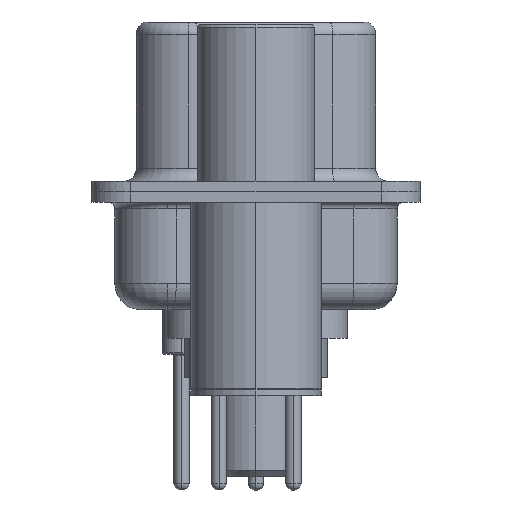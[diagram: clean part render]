
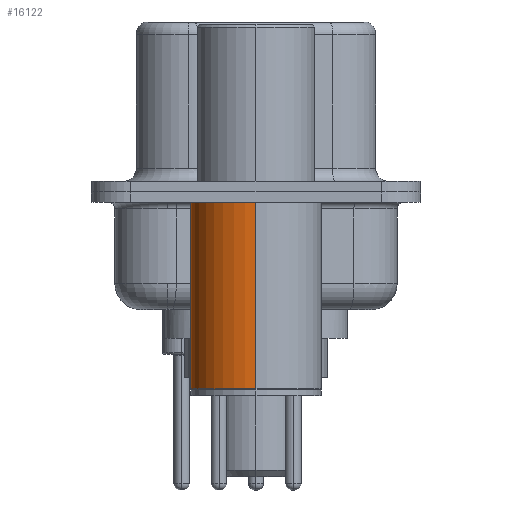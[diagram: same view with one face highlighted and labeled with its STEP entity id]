
A CAD part, left-side view. The second image highlights one B-rep face of the part: STEP entity #16122.
In plain terms, the highlighted cylindrical face has radius 2.5 mm (diameter 5 mm), a partial arc.
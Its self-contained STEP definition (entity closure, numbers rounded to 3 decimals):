
#1057 = AXIS2_PLACEMENT_3D ( 'NONE', #14917, #10517, #25536 ) ;
#2751 = CIRCLE ( 'NONE', #1057, 2.5 ) ;
#4087 = EDGE_CURVE ( 'NONE', #24441, #12162, #5364, .T. ) ;
#4224 = CARTESIAN_POINT ( 'NONE',  ( -2.5, 0., -0.4 ) ) ;
#4297 = CARTESIAN_POINT ( 'NONE',  ( 0., 0., 0.581 ) ) ;
#4834 = CYLINDRICAL_SURFACE ( 'NONE', #10473, 2.5 ) ;
#5364 = LINE ( 'NONE', #21465, #18735 ) ;
#5823 = EDGE_CURVE ( 'NONE', #15573, #17217, #18302, .T. ) ;
#6561 = DIRECTION ( 'NONE',  ( 0., 0., 1. ) ) ;
#7858 = EDGE_CURVE ( 'NONE', #12162, #17217, #18929, .T. ) ;
#8830 = ORIENTED_EDGE ( 'NONE', *, *, #5823, .T. ) ;
#9126 = CARTESIAN_POINT ( 'NONE',  ( 2.5, 0., -7.525 ) ) ;
#9498 = DIRECTION ( 'NONE',  ( 1., 0., 0. ) ) ;
#10473 = AXIS2_PLACEMENT_3D ( 'NONE', #4297, #20605, #22968 ) ;
#10517 = DIRECTION ( 'NONE',  ( 0., 0., 1. ) ) ;
#11238 = CARTESIAN_POINT ( 'NONE',  ( 2.5, 0., -0.4 ) ) ;
#11272 = VECTOR ( 'NONE', #16085, 1000. ) ;
#11969 = CARTESIAN_POINT ( 'NONE',  ( -2.5, 0., 0.581 ) ) ;
#12162 = VERTEX_POINT ( 'NONE', #11238 ) ;
#14503 = ORIENTED_EDGE ( 'NONE', *, *, #4087, .F. ) ;
#14874 = AXIS2_PLACEMENT_3D ( 'NONE', #24136, #26656, #9498 ) ;
#14917 = CARTESIAN_POINT ( 'NONE',  ( 0., 0., -7.525 ) ) ;
#15573 = VERTEX_POINT ( 'NONE', #22784 ) ;
#16085 = DIRECTION ( 'NONE',  ( 0., 0., 1. ) ) ;
#16122 = ADVANCED_FACE ( 'NONE', ( #19854 ), #4834, .T. ) ;
#17217 = VERTEX_POINT ( 'NONE', #4224 ) ;
#17948 = EDGE_CURVE ( 'NONE', #24441, #15573, #2751, .T. ) ;
#18302 = LINE ( 'NONE', #11969, #11272 ) ;
#18735 = VECTOR ( 'NONE', #6561, 1000. ) ;
#18929 = CIRCLE ( 'NONE', #14874, 2.5 ) ;
#19854 = FACE_OUTER_BOUND ( 'NONE', #22088, .T. ) ;
#20605 = DIRECTION ( 'NONE',  ( 0., 0., 1. ) ) ;
#21465 = CARTESIAN_POINT ( 'NONE',  ( 2.5, 0., 0.581 ) ) ;
#22088 = EDGE_LOOP ( 'NONE', ( #23023, #8830, #26484, #14503 ) ) ;
#22784 = CARTESIAN_POINT ( 'NONE',  ( -2.5, 0., -7.525 ) ) ;
#22968 = DIRECTION ( 'NONE',  ( 1., 0., 0. ) ) ;
#23023 = ORIENTED_EDGE ( 'NONE', *, *, #17948, .T. ) ;
#24136 = CARTESIAN_POINT ( 'NONE',  ( 0., 0., -0.4 ) ) ;
#24441 = VERTEX_POINT ( 'NONE', #9126 ) ;
#25536 = DIRECTION ( 'NONE',  ( 1., 0., 0. ) ) ;
#26484 = ORIENTED_EDGE ( 'NONE', *, *, #7858, .F. ) ;
#26656 = DIRECTION ( 'NONE',  ( 0., 0., 1. ) ) ;
